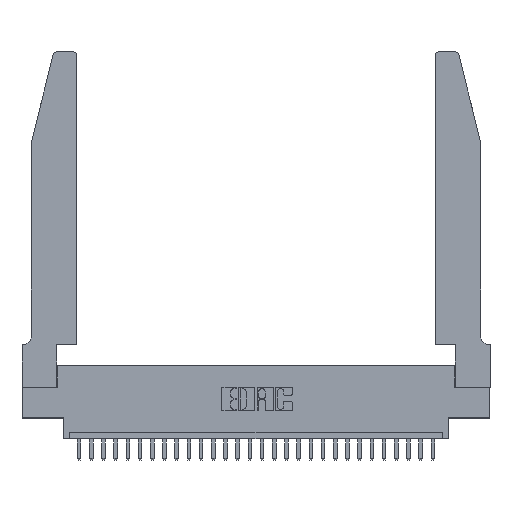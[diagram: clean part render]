
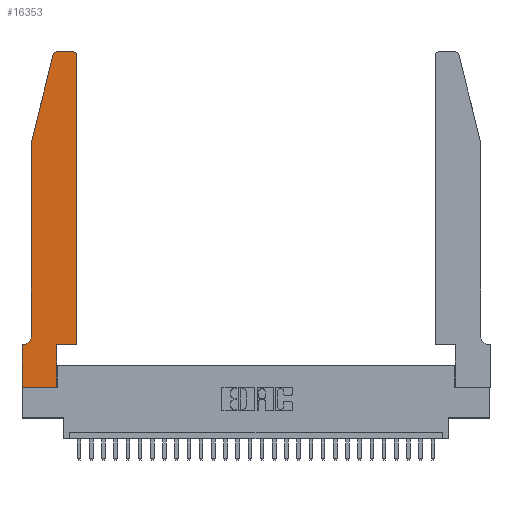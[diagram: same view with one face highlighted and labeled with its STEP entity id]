
A CAD part, top view. The second image highlights one B-rep face of the part: STEP entity #16353.
In plain terms, the highlighted planar face has unit normal (0, 0, 1).
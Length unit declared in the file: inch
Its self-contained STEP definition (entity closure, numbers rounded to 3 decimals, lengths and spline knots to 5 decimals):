
#32 = VERTEX_POINT ( 'NONE', #5507 ) ;
#269 = PLANE ( 'NONE',  #4100 ) ;
#288 = VECTOR ( 'NONE', #417, 39.37008 ) ;
#417 = DIRECTION ( 'NONE',  ( -0.239, -0.971, 0. ) ) ;
#681 = EDGE_CURVE ( 'NONE', #32, #5778, #11966, .T. ) ;
#898 = CARTESIAN_POINT ( 'NONE',  ( 0.0755, 2., 0.37 ) ) ;
#1907 = VERTEX_POINT ( 'NONE', #2625 ) ;
#2277 = EDGE_CURVE ( 'NONE', #23716, #32, #13942, .T. ) ;
#2292 = CARTESIAN_POINT ( 'NONE',  ( 0.2605, 2.75, 0.37 ) ) ;
#2530 = EDGE_CURVE ( 'NONE', #28229, #3203, #7622, .T. ) ;
#2625 = CARTESIAN_POINT ( 'NONE',  ( 0., 0.35, 0.37 ) ) ;
#2644 = VECTOR ( 'NONE', #19994, 39.37008 ) ;
#2820 = DIRECTION ( 'NONE',  ( 0., 0., 1. ) ) ;
#3194 = DIRECTION ( 'NONE',  ( 1., 0., 0. ) ) ;
#3203 = VERTEX_POINT ( 'NONE', #4540 ) ;
#3398 = EDGE_CURVE ( 'NONE', #25221, #1907, #26997, .T. ) ;
#3662 = CARTESIAN_POINT ( 'NONE',  ( 0., 0., 0.37 ) ) ;
#3665 = CARTESIAN_POINT ( 'NONE',  ( 0.4505, 0.35, 0.37 ) ) ;
#4023 = CARTESIAN_POINT ( 'NONE',  ( 0.0055, 0.35, 0.37 ) ) ;
#4100 = AXIS2_PLACEMENT_3D ( 'NONE', #20611, #2820, #7053 ) ;
#4176 = DIRECTION ( 'NONE',  ( -1., 0., 0. ) ) ;
#4540 = CARTESIAN_POINT ( 'NONE',  ( 0.0755, 0.42, 0.37 ) ) ;
#5332 = CARTESIAN_POINT ( 'NONE',  ( 0.0755, 2., 0.37 ) ) ;
#5507 = CARTESIAN_POINT ( 'NONE',  ( 0.284, 2.75, 0.37 ) ) ;
#5778 = VERTEX_POINT ( 'NONE', #8034 ) ;
#5990 = DIRECTION ( 'NONE',  ( 0., -1., 0. ) ) ;
#6156 = CARTESIAN_POINT ( 'NONE',  ( 0.0755, 0.35, 0.37 ) ) ;
#6296 = LINE ( 'NONE', #5332, #288 ) ;
#6769 = EDGE_CURVE ( 'NONE', #3203, #25221, #7773, .T. ) ;
#6931 = EDGE_CURVE ( 'NONE', #7192, #10997, #9897, .T. ) ;
#7053 = DIRECTION ( 'NONE',  ( 1., 0., 0. ) ) ;
#7173 = CARTESIAN_POINT ( 'NONE',  ( 0.0755, 2., 0.37 ) ) ;
#7192 = VERTEX_POINT ( 'NONE', #17818 ) ;
#7284 = AXIS2_PLACEMENT_3D ( 'NONE', #18400, #27369, #3194 ) ;
#7622 = LINE ( 'NONE', #7173, #22785 ) ;
#7773 = CIRCLE ( 'NONE', #15390, 0.07 ) ;
#7989 = DIRECTION ( 'NONE',  ( 0., -1., 0. ) ) ;
#8034 = CARTESIAN_POINT ( 'NONE',  ( 0.25487, 2.72718, 0.37 ) ) ;
#8925 = ORIENTED_EDGE ( 'NONE', *, *, #27899, .T. ) ;
#9220 = ORIENTED_EDGE ( 'NONE', *, *, #2530, .T. ) ;
#9272 = VECTOR ( 'NONE', #12943, 39.37008 ) ;
#9350 = DIRECTION ( 'NONE',  ( 1., 0., 0. ) ) ;
#9723 = ORIENTED_EDGE ( 'NONE', *, *, #6769, .T. ) ;
#9897 = LINE ( 'NONE', #3665, #21927 ) ;
#10997 = VERTEX_POINT ( 'NONE', #21106 ) ;
#11094 = CARTESIAN_POINT ( 'NONE',  ( 0.284, 2.72, 0.37 ) ) ;
#11201 = DIRECTION ( 'NONE',  ( 0., 0., -1. ) ) ;
#11966 = CIRCLE ( 'NONE', #14899, 0.03 ) ;
#12411 = CARTESIAN_POINT ( 'NONE',  ( 0.2865, 0.35, 0.37 ) ) ;
#12426 = CARTESIAN_POINT ( 'NONE',  ( 0., 0., 0.37 ) ) ;
#12906 = VECTOR ( 'NONE', #18574, 39.37008 ) ;
#12943 = DIRECTION ( 'NONE',  ( 1., 0., 0. ) ) ;
#13942 = LINE ( 'NONE', #2292, #12906 ) ;
#14822 = DIRECTION ( 'NONE',  ( 0., 1., 0. ) ) ;
#14899 = AXIS2_PLACEMENT_3D ( 'NONE', #11094, #18340, #9350 ) ;
#14981 = CARTESIAN_POINT ( 'NONE',  ( 0.4505, 0.35, 0.37 ) ) ;
#15390 = AXIS2_PLACEMENT_3D ( 'NONE', #29139, #11201, #4176 ) ;
#15510 = VECTOR ( 'NONE', #18272, 39.37008 ) ;
#16353 = ADVANCED_FACE ( 'NONE', ( #17089 ), #269, .T. ) ;
#17089 = FACE_OUTER_BOUND ( 'NONE', #27139, .T. ) ;
#17273 = LINE ( 'NONE', #14981, #28564 ) ;
#17634 = EDGE_CURVE ( 'NONE', #10997, #23716, #26963, .T. ) ;
#17758 = CARTESIAN_POINT ( 'NONE',  ( 0.4205, 2.75, 0.37 ) ) ;
#17818 = CARTESIAN_POINT ( 'NONE',  ( 0.4505, 0.35, 0.37 ) ) ;
#18272 = DIRECTION ( 'NONE',  ( 0., 1., 0. ) ) ;
#18335 = ORIENTED_EDGE ( 'NONE', *, *, #3398, .T. ) ;
#18340 = DIRECTION ( 'NONE',  ( 0., 0., 1. ) ) ;
#18400 = CARTESIAN_POINT ( 'NONE',  ( 0.4205, 2.72, 0.37 ) ) ;
#18574 = DIRECTION ( 'NONE',  ( -1., 0., 0. ) ) ;
#19322 = ORIENTED_EDGE ( 'NONE', *, *, #17634, .T. ) ;
#19994 = DIRECTION ( 'NONE',  ( -1., 0., 0. ) ) ;
#20105 = ORIENTED_EDGE ( 'NONE', *, *, #6931, .T. ) ;
#20611 = CARTESIAN_POINT ( 'NONE',  ( 0., 0.35, 0.37 ) ) ;
#21106 = CARTESIAN_POINT ( 'NONE',  ( 0.4505, 2.72, 0.37 ) ) ;
#21261 = VERTEX_POINT ( 'NONE', #28734 ) ;
#21267 = ORIENTED_EDGE ( 'NONE', *, *, #28111, .T. ) ;
#21268 = LINE ( 'NONE', #12426, #23738 ) ;
#21895 = ORIENTED_EDGE ( 'NONE', *, *, #23323, .T. ) ;
#21927 = VECTOR ( 'NONE', #14822, 39.37008 ) ;
#21941 = ORIENTED_EDGE ( 'NONE', *, *, #681, .T. ) ;
#21987 = DIRECTION ( 'NONE',  ( 1., 0., 0. ) ) ;
#22181 = ORIENTED_EDGE ( 'NONE', *, *, #22929, .T. ) ;
#22523 = CARTESIAN_POINT ( 'NONE',  ( 0.2865, 0.35, 0.37 ) ) ;
#22785 = VECTOR ( 'NONE', #5990, 39.37008 ) ;
#22929 = EDGE_CURVE ( 'NONE', #21261, #27058, #28738, .T. ) ;
#23323 = EDGE_CURVE ( 'NONE', #1907, #21261, #21268, .T. ) ;
#23716 = VERTEX_POINT ( 'NONE', #17758 ) ;
#23738 = VECTOR ( 'NONE', #7989, 39.37008 ) ;
#23793 = ORIENTED_EDGE ( 'NONE', *, *, #25058, .T. ) ;
#23990 = ORIENTED_EDGE ( 'NONE', *, *, #2277, .T. ) ;
#24974 = VERTEX_POINT ( 'NONE', #12411 ) ;
#25058 = EDGE_CURVE ( 'NONE', #24974, #7192, #17273, .T. ) ;
#25221 = VERTEX_POINT ( 'NONE', #4023 ) ;
#26963 = CIRCLE ( 'NONE', #7284, 0.03 ) ;
#26997 = LINE ( 'NONE', #6156, #2644 ) ;
#27058 = VERTEX_POINT ( 'NONE', #28193 ) ;
#27139 = EDGE_LOOP ( 'NONE', ( #23990, #21941, #21267, #9220, #9723, #18335, #21895, #22181, #8925, #23793, #20105, #19322 ) ) ;
#27369 = DIRECTION ( 'NONE',  ( 0., 0., 1. ) ) ;
#27501 = LINE ( 'NONE', #22523, #15510 ) ;
#27899 = EDGE_CURVE ( 'NONE', #27058, #24974, #27501, .T. ) ;
#28111 = EDGE_CURVE ( 'NONE', #5778, #28229, #6296, .T. ) ;
#28193 = CARTESIAN_POINT ( 'NONE',  ( 0.2865, 0., 0.37 ) ) ;
#28229 = VERTEX_POINT ( 'NONE', #898 ) ;
#28564 = VECTOR ( 'NONE', #21987, 39.37008 ) ;
#28734 = CARTESIAN_POINT ( 'NONE',  ( 0., 0., 0.37 ) ) ;
#28738 = LINE ( 'NONE', #3662, #9272 ) ;
#29139 = CARTESIAN_POINT ( 'NONE',  ( 0.0055, 0.42, 0.37 ) ) ;
